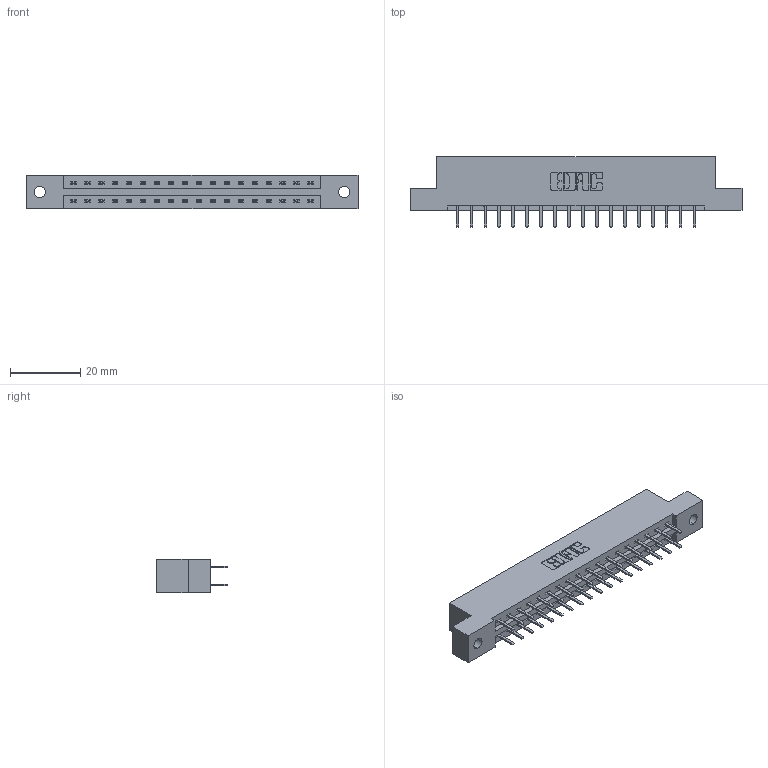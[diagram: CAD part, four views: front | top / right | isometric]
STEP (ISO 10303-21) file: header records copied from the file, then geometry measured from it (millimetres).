
FILE_DESCRIPTION (( 'STEP AP203' ), '1' );
FILE_NAME ('387-036-520-202.STEP', '2018-09-18T23:08:28', ( '' ), ( '' ), 'SwSTEP 2.0', 'SolidWorks 2016', '' );
FILE_SCHEMA (( 'CONFIG_CONTROL_DESIGN' ));
Length unit declared in the file: inch
Products named in the file (3): 337 Part_Flush Mounting Lugs - 0.128 Dia; 345-292-001_345-293-120; 387-036-520-202
Assembly tree (37 placements, depth 2):
  387-036-520-202
    337 Part_Flush Mounting Lugs - 0.128 Dia
    345-292-001_345-293-120  x36
Bounding box: 94.34 x 20.02 x 9.4 mm (x, y, z)
Volume: 9569.9 mm3; surface area: 10267.8 mm2
Topology: 37 solids, 37 shells, 2202 faces, 6395 edges, 4166 vertices
Faces by surface type: plane 1510, cylinder 692
Entity records: 17177 total; most frequent: CARTESIAN_POINT 2926, ORIENTED_EDGE 2850, DIRECTION 2521, EDGE_CURVE 1425, VECTOR 1293, LINE 1293, VERTEX_POINT 946, AXIS2_PLACEMENT_3D 614
